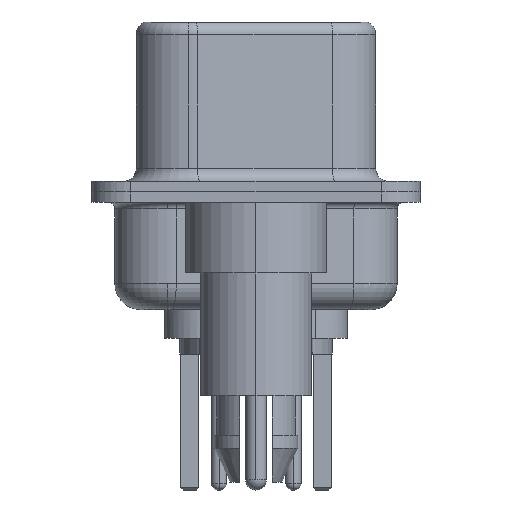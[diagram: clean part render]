
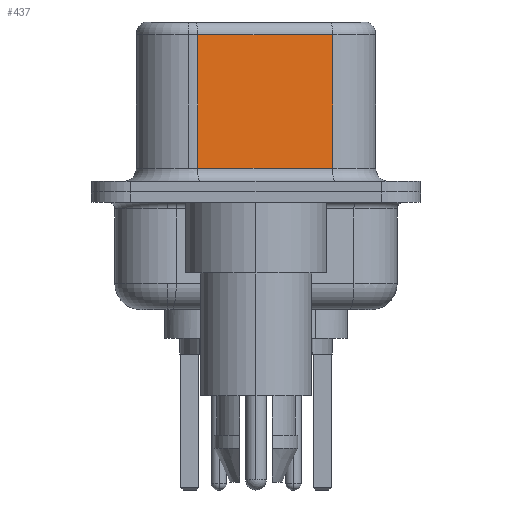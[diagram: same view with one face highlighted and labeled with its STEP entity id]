
A CAD part, left-side view. The second image highlights one B-rep face of the part: STEP entity #437.
In plain terms, the highlighted planar face has unit normal (-0.985, -0.174, 0).
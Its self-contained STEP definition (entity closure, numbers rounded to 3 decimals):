
#437 = ADVANCED_FACE ( 'NONE', ( #6553 ), #4179, .F. ) ;
#535 = DIRECTION ( 'NONE',  ( 0.985, 0.174, 0. ) ) ;
#778 = DIRECTION ( 'NONE',  ( 0., 0., -1. ) ) ;
#826 = EDGE_CURVE ( 'NONE', #5987, #11826, #1060, .T. ) ;
#1060 = LINE ( 'NONE', #2498, #5541 ) ;
#1799 = VECTOR ( 'NONE', #778, 1000. ) ;
#1805 = CARTESIAN_POINT ( 'NONE',  ( 3.67, 2.233, 0.9 ) ) ;
#2498 = CARTESIAN_POINT ( 'NONE',  ( 4.58, -2.927, 0.9 ) ) ;
#3474 = EDGE_LOOP ( 'NONE', ( #10106, #5007, #3620, #10061 ) ) ;
#3494 = DIRECTION ( 'NONE',  ( 0.174, -0.985, 0. ) ) ;
#3620 = ORIENTED_EDGE ( 'NONE', *, *, #18786, .T. ) ;
#3812 = DIRECTION ( 'NONE',  ( 0., 0., -1. ) ) ;
#4179 = PLANE ( 'NONE',  #14305 ) ;
#4525 = CARTESIAN_POINT ( 'NONE',  ( 4.58, -2.927, 6.02 ) ) ;
#5007 = ORIENTED_EDGE ( 'NONE', *, *, #19733, .T. ) ;
#5541 = VECTOR ( 'NONE', #3494, 1000. ) ;
#5987 = VERTEX_POINT ( 'NONE', #1805 ) ;
#6268 = LINE ( 'NONE', #10811, #1799 ) ;
#6317 = DIRECTION ( 'NONE',  ( -0.174, 0.985, 0. ) ) ;
#6553 = FACE_OUTER_BOUND ( 'NONE', #3474, .T. ) ;
#8231 = CARTESIAN_POINT ( 'NONE',  ( 3.67, 2.233, 6.02 ) ) ;
#8774 = LINE ( 'NONE', #13851, #9290 ) ;
#9085 = DIRECTION ( 'NONE',  ( -0.174, 0.985, 0. ) ) ;
#9290 = VECTOR ( 'NONE', #3812, 1000. ) ;
#9589 = CARTESIAN_POINT ( 'NONE',  ( 4.58, -2.927, 6.02 ) ) ;
#10061 = ORIENTED_EDGE ( 'NONE', *, *, #826, .T. ) ;
#10106 = ORIENTED_EDGE ( 'NONE', *, *, #16437, .F. ) ;
#10775 = CARTESIAN_POINT ( 'NONE',  ( 4.58, -2.927, 6.52 ) ) ;
#10811 = CARTESIAN_POINT ( 'NONE',  ( 4.58, -2.927, 6.52 ) ) ;
#11350 = VECTOR ( 'NONE', #6317, 1000. ) ;
#11826 = VERTEX_POINT ( 'NONE', #17165 ) ;
#12806 = VERTEX_POINT ( 'NONE', #8231 ) ;
#13851 = CARTESIAN_POINT ( 'NONE',  ( 3.67, 2.233, 6.52 ) ) ;
#14305 = AXIS2_PLACEMENT_3D ( 'NONE', #10775, #535, #9085 ) ;
#14942 = VERTEX_POINT ( 'NONE', #4525 ) ;
#16437 = EDGE_CURVE ( 'NONE', #14942, #11826, #6268, .T. ) ;
#17165 = CARTESIAN_POINT ( 'NONE',  ( 4.58, -2.927, 0.9 ) ) ;
#18786 = EDGE_CURVE ( 'NONE', #12806, #5987, #8774, .T. ) ;
#19733 = EDGE_CURVE ( 'NONE', #14942, #12806, #20289, .T. ) ;
#20289 = LINE ( 'NONE', #9589, #11350 ) ;
